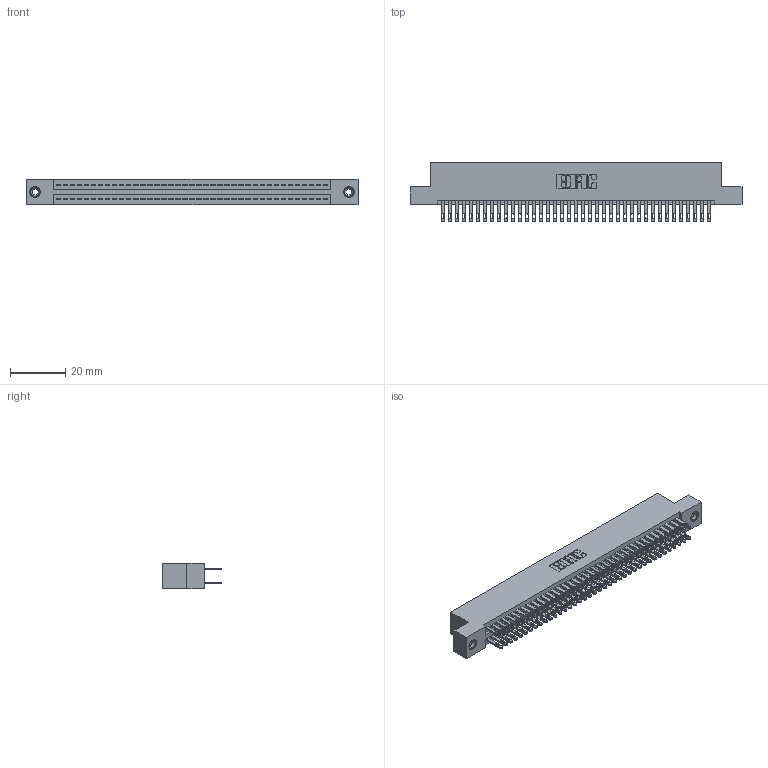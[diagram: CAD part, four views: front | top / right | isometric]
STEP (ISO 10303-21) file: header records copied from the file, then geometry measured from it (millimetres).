
FILE_DESCRIPTION (( 'STEP AP203' ), '1' );
FILE_NAME ('345-078-500-208.STEP', '2018-10-02T18:57:55', ( '' ), ( '' ), 'SwSTEP 2.0', 'SolidWorks 2016', '' );
FILE_SCHEMA (( 'CONFIG_CONTROL_DESIGN' ));
Length unit declared in the file: inch
Products named in the file (4): 345-292-001_345-293-100; 345 Part_Flush Mounting Lugs - 0.156 Dia-TI; 345-078-500-208; 345-250-001_345-250-003-102
Assembly tree (81 placements, depth 2):
  345-078-500-208
    345 Part_Flush Mounting Lugs - 0.156 Dia-TI
    345-292-001_345-293-100  x78
    345-250-001_345-250-003-102  x2
Bounding box: 120.27 x 21.51 x 9.4 mm (x, y, z)
Volume: 11887 mm3; surface area: 18321.9 mm2
Topology: 81 solids, 81 shells, 3774 faces, 11475 edges, 7642 vertices
Faces by surface type: plane 2218, cylinder 1540, cone 12, torus 4
Entity records: 32120 total; most frequent: CARTESIAN_POINT 5367, ORIENTED_EDGE 5294, DIRECTION 4765, EDGE_CURVE 2647, LINE 2335, VECTOR 2335, VERTEX_POINT 1760, AXIS2_PLACEMENT_3D 1215
